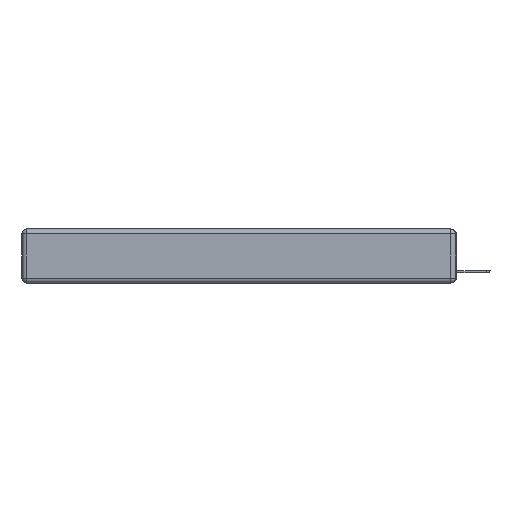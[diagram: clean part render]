
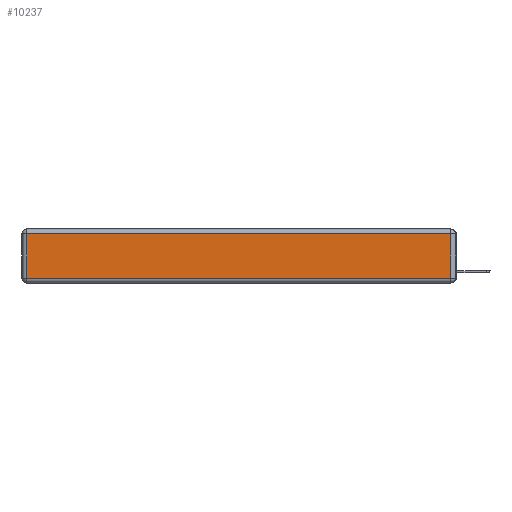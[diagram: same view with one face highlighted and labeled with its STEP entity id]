
A CAD part, left-side view. The second image highlights one B-rep face of the part: STEP entity #10237.
In plain terms, the highlighted planar face has unit normal (-1, 0, 0).
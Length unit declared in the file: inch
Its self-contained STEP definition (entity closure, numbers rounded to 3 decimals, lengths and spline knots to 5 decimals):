
#335 = EDGE_CURVE ( 'NONE', #10795, #1287, #15562, .T. ) ;
#419 = CARTESIAN_POINT ( 'NONE',  ( 0., 2.75, -0.03 ) ) ;
#1061 = EDGE_CURVE ( 'NONE', #9324, #10795, #7879, .T. ) ;
#1155 = ORIENTED_EDGE ( 'NONE', *, *, #4045, .T. ) ;
#1287 = VERTEX_POINT ( 'NONE', #7831 ) ;
#1815 = VECTOR ( 'NONE', #17775, 39.37008 ) ;
#2943 = VECTOR ( 'NONE', #19609, 39.37008 ) ;
#4045 = EDGE_CURVE ( 'NONE', #20036, #9324, #9969, .T. ) ;
#6129 = CARTESIAN_POINT ( 'NONE',  ( 0., 0.03, -0.343 ) ) ;
#6636 = FACE_OUTER_BOUND ( 'NONE', #18202, .T. ) ;
#7005 = DIRECTION ( 'NONE',  ( 0., 0., 1. ) ) ;
#7459 = DIRECTION ( 'NONE',  ( 0., -1., 0. ) ) ;
#7479 = AXIS2_PLACEMENT_3D ( 'NONE', #8654, #18084, #7005 ) ;
#7831 = CARTESIAN_POINT ( 'NONE',  ( 0., 0.03, -0.313 ) ) ;
#7879 = LINE ( 'NONE', #11769, #2943 ) ;
#8495 = CARTESIAN_POINT ( 'NONE',  ( 0., 2.72, -0.313 ) ) ;
#8654 = CARTESIAN_POINT ( 'NONE',  ( 0., 0., -0.343 ) ) ;
#9324 = VERTEX_POINT ( 'NONE', #15071 ) ;
#9969 = LINE ( 'NONE', #419, #1815 ) ;
#10237 = ADVANCED_FACE ( 'NONE', ( #6636 ), #13193, .T. ) ;
#10755 = ORIENTED_EDGE ( 'NONE', *, *, #1061, .T. ) ;
#10795 = VERTEX_POINT ( 'NONE', #8495 ) ;
#11769 = CARTESIAN_POINT ( 'NONE',  ( 0., 2.72, -0.343 ) ) ;
#13163 = CARTESIAN_POINT ( 'NONE',  ( 0., 0.03, -0.03 ) ) ;
#13193 = PLANE ( 'NONE',  #7479 ) ;
#13952 = ORIENTED_EDGE ( 'NONE', *, *, #335, .T. ) ;
#14918 = EDGE_CURVE ( 'NONE', #1287, #20036, #17313, .T. ) ;
#15071 = CARTESIAN_POINT ( 'NONE',  ( 0., 2.72, -0.03 ) ) ;
#15562 = LINE ( 'NONE', #18736, #18748 ) ;
#16518 = ORIENTED_EDGE ( 'NONE', *, *, #14918, .T. ) ;
#16819 = VECTOR ( 'NONE', #20111, 39.37008 ) ;
#17313 = LINE ( 'NONE', #6129, #16819 ) ;
#17775 = DIRECTION ( 'NONE',  ( 0., 1., 0. ) ) ;
#18084 = DIRECTION ( 'NONE',  ( -1., 0., 0. ) ) ;
#18202 = EDGE_LOOP ( 'NONE', ( #13952, #16518, #1155, #10755 ) ) ;
#18736 = CARTESIAN_POINT ( 'NONE',  ( 0., 0., -0.313 ) ) ;
#18748 = VECTOR ( 'NONE', #7459, 39.37008 ) ;
#19609 = DIRECTION ( 'NONE',  ( 0., 0., -1. ) ) ;
#20036 = VERTEX_POINT ( 'NONE', #13163 ) ;
#20111 = DIRECTION ( 'NONE',  ( 0., 0., 1. ) ) ;
